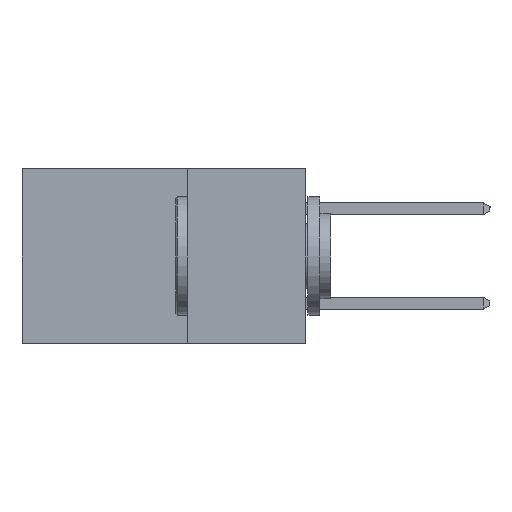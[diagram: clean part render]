
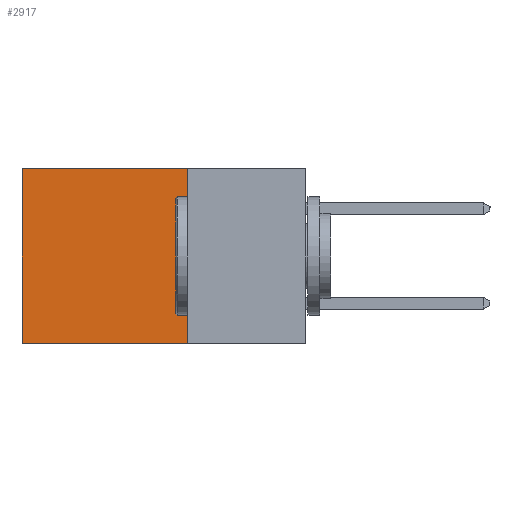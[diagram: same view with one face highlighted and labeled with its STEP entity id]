
A CAD part, left-side view. The second image highlights one B-rep face of the part: STEP entity #2917.
In plain terms, the highlighted planar face has unit normal (-1, 0, 0).
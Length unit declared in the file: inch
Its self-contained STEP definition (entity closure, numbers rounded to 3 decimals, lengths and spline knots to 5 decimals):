
#15 = CARTESIAN_POINT ( 'NONE',  ( 0.2615, 0.6, -0.37 ) ) ;
#367 = DIRECTION ( 'NONE',  ( 0., 0., -1. ) ) ;
#821 = CARTESIAN_POINT ( 'NONE',  ( 0.2615, 0.25, -0.37 ) ) ;
#1071 = DIRECTION ( 'NONE',  ( 0., 1., 0. ) ) ;
#2917 = ADVANCED_FACE ( 'NONE', ( #3625 ), #10450, .F. ) ;
#3332 = LINE ( 'NONE', #12470, #20310 ) ;
#3395 = DIRECTION ( 'NONE',  ( 1., 0., 0. ) ) ;
#3625 = FACE_OUTER_BOUND ( 'NONE', #22082, .T. ) ;
#4438 = LINE ( 'NONE', #16863, #14901 ) ;
#5706 = CARTESIAN_POINT ( 'NONE',  ( 0.2615, 0.25, 0. ) ) ;
#6068 = EDGE_CURVE ( 'NONE', #15270, #17123, #20716, .T. ) ;
#7366 = CARTESIAN_POINT ( 'NONE',  ( 0.2615, 0.25, -0.37 ) ) ;
#7717 = VERTEX_POINT ( 'NONE', #5706 ) ;
#8296 = ORIENTED_EDGE ( 'NONE', *, *, #22003, .F. ) ;
#8536 = CARTESIAN_POINT ( 'NONE',  ( 0.2615, 0.6, 0. ) ) ;
#9703 = ORIENTED_EDGE ( 'NONE', *, *, #6068, .F. ) ;
#9716 = VERTEX_POINT ( 'NONE', #8536 ) ;
#10450 = PLANE ( 'NONE',  #11944 ) ;
#11944 = AXIS2_PLACEMENT_3D ( 'NONE', #7366, #3395, #21283 ) ;
#12181 = ORIENTED_EDGE ( 'NONE', *, *, #22610, .T. ) ;
#12470 = CARTESIAN_POINT ( 'NONE',  ( 0.2615, 0.25, -0.37 ) ) ;
#12841 = CARTESIAN_POINT ( 'NONE',  ( 0.2615, 0.6, -0.37 ) ) ;
#14543 = LINE ( 'NONE', #15, #15102 ) ;
#14901 = VECTOR ( 'NONE', #16628, 39.37008 ) ;
#14954 = EDGE_CURVE ( 'NONE', #7717, #9716, #4438, .T. ) ;
#15102 = VECTOR ( 'NONE', #367, 39.37008 ) ;
#15270 = VERTEX_POINT ( 'NONE', #18256 ) ;
#16628 = DIRECTION ( 'NONE',  ( 0., 1., 0. ) ) ;
#16863 = CARTESIAN_POINT ( 'NONE',  ( 0.2615, 0.25, 0. ) ) ;
#16959 = ORIENTED_EDGE ( 'NONE', *, *, #14954, .T. ) ;
#17006 = VECTOR ( 'NONE', #1071, 39.37008 ) ;
#17123 = VERTEX_POINT ( 'NONE', #12841 ) ;
#18256 = CARTESIAN_POINT ( 'NONE',  ( 0.2615, 0.25, -0.37 ) ) ;
#20310 = VECTOR ( 'NONE', #22861, 39.37008 ) ;
#20716 = LINE ( 'NONE', #821, #17006 ) ;
#21283 = DIRECTION ( 'NONE',  ( 0., 0., -1. ) ) ;
#22003 = EDGE_CURVE ( 'NONE', #7717, #15270, #3332, .T. ) ;
#22082 = EDGE_LOOP ( 'NONE', ( #12181, #9703, #8296, #16959 ) ) ;
#22610 = EDGE_CURVE ( 'NONE', #9716, #17123, #14543, .T. ) ;
#22861 = DIRECTION ( 'NONE',  ( 0., 0., -1. ) ) ;
